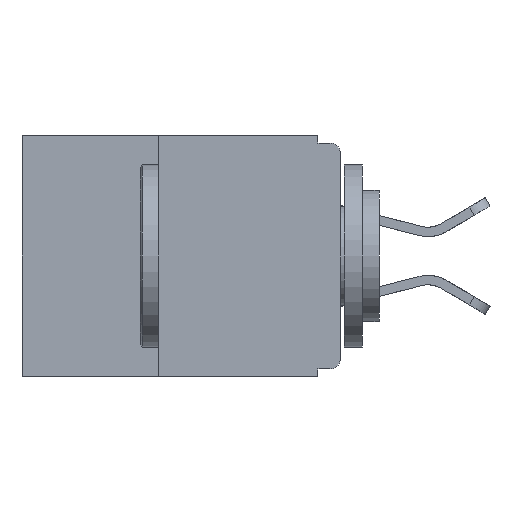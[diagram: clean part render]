
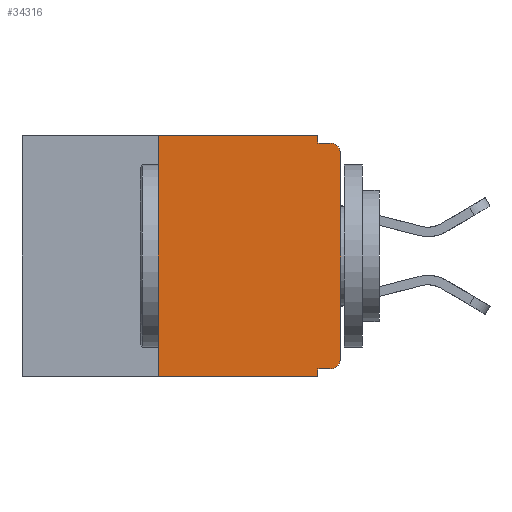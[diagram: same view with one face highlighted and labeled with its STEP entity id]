
A CAD part, left-side view. The second image highlights one B-rep face of the part: STEP entity #34316.
In plain terms, the highlighted planar face has unit normal (-1, 0, 0).
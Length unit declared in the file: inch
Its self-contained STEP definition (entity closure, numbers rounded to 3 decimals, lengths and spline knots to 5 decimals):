
#244 = VERTEX_POINT ( 'NONE', #8070 ) ;
#679 = VECTOR ( 'NONE', #13537, 39.37008 ) ;
#1655 = CARTESIAN_POINT ( 'NONE',  ( 0., 0.031, 0. ) ) ;
#1808 = CARTESIAN_POINT ( 'NONE',  ( 0., 0.015, -0.025 ) ) ;
#2243 = LINE ( 'NONE', #25269, #16544 ) ;
#2446 = VERTEX_POINT ( 'NONE', #24529 ) ;
#4247 = LINE ( 'NONE', #32721, #24964 ) ;
#4508 = DIRECTION ( 'NONE',  ( 0., 0., -1. ) ) ;
#4672 = DIRECTION ( 'NONE',  ( 0., 0., -1. ) ) ;
#4787 = CARTESIAN_POINT ( 'NONE',  ( 0., 0.015, -0.01 ) ) ;
#5308 = EDGE_LOOP ( 'NONE', ( #12681, #13550, #14452, #15131, #15528, #16009, #16043, #16630, #17586, #17653 ) ) ;
#7256 = FACE_OUTER_BOUND ( 'NONE', #5308, .T. ) ;
#7638 = CARTESIAN_POINT ( 'NONE',  ( 0., 0., -0.305 ) ) ;
#7880 = DIRECTION ( 'NONE',  ( 1., 0., 0. ) ) ;
#8070 = CARTESIAN_POINT ( 'NONE',  ( 0., 0.25, -0.33 ) ) ;
#8439 = EDGE_CURVE ( 'NONE', #10893, #29079, #32629, .T. ) ;
#8655 = AXIS2_PLACEMENT_3D ( 'NONE', #1808, #21660, #4672 ) ;
#8865 = AXIS2_PLACEMENT_3D ( 'NONE', #11399, #30899, #14291 ) ;
#9154 = CARTESIAN_POINT ( 'NONE',  ( 0., 0., -0.025 ) ) ;
#9287 = EDGE_CURVE ( 'NONE', #25720, #12900, #23724, .T. ) ;
#10108 = LINE ( 'NONE', #27763, #30608 ) ;
#10893 = VERTEX_POINT ( 'NONE', #18510 ) ;
#11240 = CARTESIAN_POINT ( 'NONE',  ( 0., 0.437, 0. ) ) ;
#11399 = CARTESIAN_POINT ( 'NONE',  ( 0., 0.015, -0.305 ) ) ;
#12559 = DIRECTION ( 'NONE',  ( 0., 0., 1. ) ) ;
#12681 = ORIENTED_EDGE ( 'NONE', *, *, #23876, .T. ) ;
#12900 = VERTEX_POINT ( 'NONE', #7638 ) ;
#13537 = DIRECTION ( 'NONE',  ( 0., -1., 0. ) ) ;
#13550 = ORIENTED_EDGE ( 'NONE', *, *, #26036, .T. ) ;
#13582 = LINE ( 'NONE', #11240, #21044 ) ;
#14059 = CARTESIAN_POINT ( 'NONE',  ( 0., 0.031, -0.33 ) ) ;
#14241 = VERTEX_POINT ( 'NONE', #23049 ) ;
#14291 = DIRECTION ( 'NONE',  ( 0., 0., -1. ) ) ;
#14452 = ORIENTED_EDGE ( 'NONE', *, *, #8439, .F. ) ;
#14609 = CARTESIAN_POINT ( 'NONE',  ( 0., 0.015, -0.32 ) ) ;
#15131 = ORIENTED_EDGE ( 'NONE', *, *, #19258, .F. ) ;
#15528 = ORIENTED_EDGE ( 'NONE', *, *, #21209, .F. ) ;
#16009 = ORIENTED_EDGE ( 'NONE', *, *, #19311, .F. ) ;
#16043 = ORIENTED_EDGE ( 'NONE', *, *, #26687, .T. ) ;
#16213 = VECTOR ( 'NONE', #25760, 39.37008 ) ;
#16544 = VECTOR ( 'NONE', #28070, 39.37008 ) ;
#16630 = ORIENTED_EDGE ( 'NONE', *, *, #23022, .F. ) ;
#17586 = ORIENTED_EDGE ( 'NONE', *, *, #26204, .F. ) ;
#17653 = ORIENTED_EDGE ( 'NONE', *, *, #9287, .T. ) ;
#18510 = CARTESIAN_POINT ( 'NONE',  ( 0., 0.031, -0.01 ) ) ;
#18961 = VERTEX_POINT ( 'NONE', #25569 ) ;
#19258 = EDGE_CURVE ( 'NONE', #18961, #10893, #20291, .T. ) ;
#19311 = EDGE_CURVE ( 'NONE', #244, #14241, #4247, .T. ) ;
#20291 = LINE ( 'NONE', #1655, #34054 ) ;
#21044 = VECTOR ( 'NONE', #27967, 39.37008 ) ;
#21209 = EDGE_CURVE ( 'NONE', #14241, #18961, #13582, .T. ) ;
#21660 = DIRECTION ( 'NONE',  ( -1., 0., 0. ) ) ;
#22996 = CARTESIAN_POINT ( 'NONE',  ( 0., 0., -0.01 ) ) ;
#23022 = EDGE_CURVE ( 'NONE', #2446, #26256, #2243, .T. ) ;
#23049 = CARTESIAN_POINT ( 'NONE',  ( 0., 0.25, 0. ) ) ;
#23204 = LINE ( 'NONE', #35518, #679 ) ;
#23436 = AXIS2_PLACEMENT_3D ( 'NONE', #24676, #7880, #27484 ) ;
#23724 = CIRCLE ( 'NONE', #8865, 0.015 ) ;
#23876 = EDGE_CURVE ( 'NONE', #12900, #26995, #32910, .T. ) ;
#24529 = CARTESIAN_POINT ( 'NONE',  ( 0., 0.031, -0.32 ) ) ;
#24676 = CARTESIAN_POINT ( 'NONE',  ( 0., 0.437, 0. ) ) ;
#24964 = VECTOR ( 'NONE', #29915, 39.37008 ) ;
#25269 = CARTESIAN_POINT ( 'NONE',  ( 0., 0.031, -0.33 ) ) ;
#25569 = CARTESIAN_POINT ( 'NONE',  ( 0., 0.031, 0. ) ) ;
#25720 = VERTEX_POINT ( 'NONE', #14609 ) ;
#25760 = DIRECTION ( 'NONE',  ( 0., -1., 0. ) ) ;
#26036 = EDGE_CURVE ( 'NONE', #26995, #29079, #29325, .T. ) ;
#26204 = EDGE_CURVE ( 'NONE', #25720, #2446, #10108, .T. ) ;
#26256 = VERTEX_POINT ( 'NONE', #14059 ) ;
#26407 = CARTESIAN_POINT ( 'NONE',  ( 0., 0., 0. ) ) ;
#26687 = EDGE_CURVE ( 'NONE', #244, #26256, #23204, .T. ) ;
#26995 = VERTEX_POINT ( 'NONE', #9154 ) ;
#27484 = DIRECTION ( 'NONE',  ( 0., 0., -1. ) ) ;
#27763 = CARTESIAN_POINT ( 'NONE',  ( 0., 0., -0.32 ) ) ;
#27967 = DIRECTION ( 'NONE',  ( 0., -1., 0. ) ) ;
#28070 = DIRECTION ( 'NONE',  ( 0., 0., -1. ) ) ;
#29079 = VERTEX_POINT ( 'NONE', #4787 ) ;
#29325 = CIRCLE ( 'NONE', #8655, 0.015 ) ;
#29915 = DIRECTION ( 'NONE',  ( 0., 0., 1. ) ) ;
#30553 = DIRECTION ( 'NONE',  ( 0., 1., 0. ) ) ;
#30608 = VECTOR ( 'NONE', #30553, 39.37008 ) ;
#30899 = DIRECTION ( 'NONE',  ( -1., 0., 0. ) ) ;
#31170 = VECTOR ( 'NONE', #12559, 39.37008 ) ;
#32629 = LINE ( 'NONE', #22996, #16213 ) ;
#32721 = CARTESIAN_POINT ( 'NONE',  ( 0., 0.25, -0.33 ) ) ;
#32910 = LINE ( 'NONE', #26407, #31170 ) ;
#34054 = VECTOR ( 'NONE', #4508, 39.37008 ) ;
#34316 = ADVANCED_FACE ( 'NONE', ( #7256 ), #35615, .F. ) ;
#35518 = CARTESIAN_POINT ( 'NONE',  ( 0., 0.437, -0.33 ) ) ;
#35615 = PLANE ( 'NONE',  #23436 ) ;
